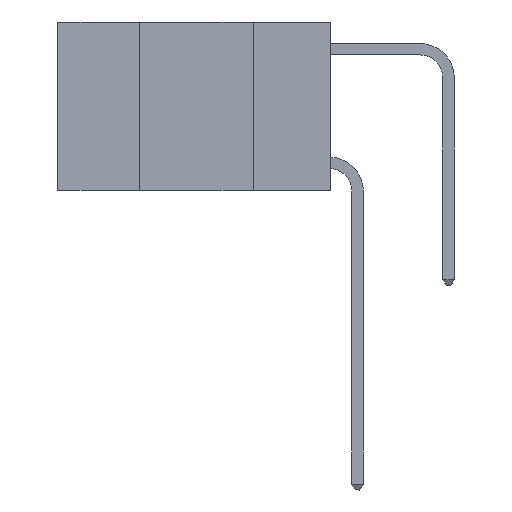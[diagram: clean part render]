
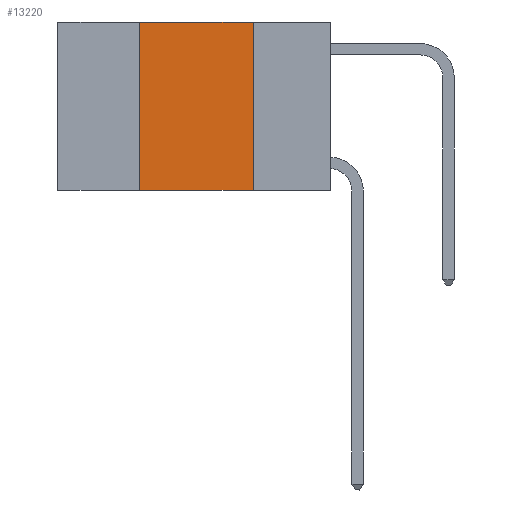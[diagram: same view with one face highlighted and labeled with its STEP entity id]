
A CAD part, left-side view. The second image highlights one B-rep face of the part: STEP entity #13220.
In plain terms, the highlighted planar face has unit normal (-1, 0, 0).
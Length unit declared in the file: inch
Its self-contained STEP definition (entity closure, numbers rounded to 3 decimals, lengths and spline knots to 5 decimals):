
#1655 = CARTESIAN_POINT ( 'NONE',  ( 0., 0.42, 0. ) ) ;
#1824 = DIRECTION ( 'NONE',  ( 0., -1., 0. ) ) ;
#2061 = VECTOR ( 'NONE', #25437, 39.37008 ) ;
#2286 = CARTESIAN_POINT ( 'NONE',  ( 0., 0.6, 0. ) ) ;
#2375 = CARTESIAN_POINT ( 'NONE',  ( 0., 0.17, 0. ) ) ;
#2448 = VECTOR ( 'NONE', #3982, 39.37008 ) ;
#3308 = ORIENTED_EDGE ( 'NONE', *, *, #4316, .F. ) ;
#3605 = CARTESIAN_POINT ( 'NONE',  ( 0., 0.17, -0.37 ) ) ;
#3982 = DIRECTION ( 'NONE',  ( 0., 0., 1. ) ) ;
#4316 = EDGE_CURVE ( 'NONE', #24608, #19866, #8393, .T. ) ;
#6134 = LINE ( 'NONE', #2375, #6795 ) ;
#6795 = VECTOR ( 'NONE', #17221, 39.37008 ) ;
#8393 = LINE ( 'NONE', #10586, #2061 ) ;
#8714 = DIRECTION ( 'NONE',  ( 1., 0., 0. ) ) ;
#10318 = CARTESIAN_POINT ( 'NONE',  ( 0., 0.42, 0. ) ) ;
#10586 = CARTESIAN_POINT ( 'NONE',  ( 0., 0.6, 0. ) ) ;
#12402 = CARTESIAN_POINT ( 'NONE',  ( 0., 0.6, -0.37 ) ) ;
#12861 = PLANE ( 'NONE',  #15963 ) ;
#13066 = EDGE_CURVE ( 'NONE', #17015, #21234, #23476, .T. ) ;
#13220 = ADVANCED_FACE ( 'NONE', ( #14543 ), #12861, .F. ) ;
#13952 = ORIENTED_EDGE ( 'NONE', *, *, #25297, .F. ) ;
#14393 = LINE ( 'NONE', #10318, #2448 ) ;
#14543 = FACE_OUTER_BOUND ( 'NONE', #15238, .T. ) ;
#15238 = EDGE_LOOP ( 'NONE', ( #13952, #3308, #15259, #26521 ) ) ;
#15259 = ORIENTED_EDGE ( 'NONE', *, *, #18755, .F. ) ;
#15963 = AXIS2_PLACEMENT_3D ( 'NONE', #2286, #8714, #23493 ) ;
#17015 = VERTEX_POINT ( 'NONE', #24150 ) ;
#17221 = DIRECTION ( 'NONE',  ( 0., 0., -1. ) ) ;
#17880 = VECTOR ( 'NONE', #1824, 39.37008 ) ;
#18585 = CARTESIAN_POINT ( 'NONE',  ( 0., 0.17, 0. ) ) ;
#18755 = EDGE_CURVE ( 'NONE', #17015, #24608, #14393, .T. ) ;
#19866 = VERTEX_POINT ( 'NONE', #18585 ) ;
#21234 = VERTEX_POINT ( 'NONE', #3605 ) ;
#23476 = LINE ( 'NONE', #12402, #17880 ) ;
#23493 = DIRECTION ( 'NONE',  ( 0., 0., -1. ) ) ;
#24150 = CARTESIAN_POINT ( 'NONE',  ( 0., 0.42, -0.37 ) ) ;
#24608 = VERTEX_POINT ( 'NONE', #1655 ) ;
#25297 = EDGE_CURVE ( 'NONE', #19866, #21234, #6134, .T. ) ;
#25437 = DIRECTION ( 'NONE',  ( 0., -1., 0. ) ) ;
#26521 = ORIENTED_EDGE ( 'NONE', *, *, #13066, .T. ) ;
